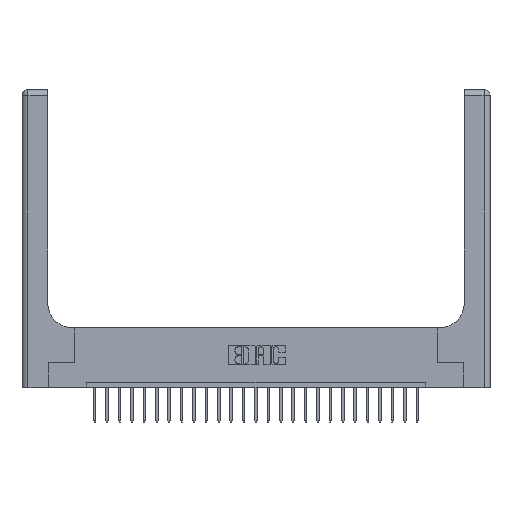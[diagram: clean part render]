
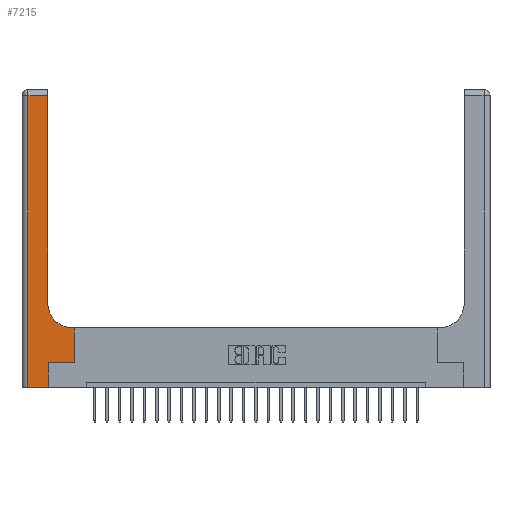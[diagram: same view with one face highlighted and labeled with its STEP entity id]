
A CAD part, top view. The second image highlights one B-rep face of the part: STEP entity #7215.
In plain terms, the highlighted planar face has unit normal (0, 0, 1).
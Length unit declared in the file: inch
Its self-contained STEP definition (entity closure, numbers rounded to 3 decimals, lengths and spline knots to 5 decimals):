
#197 = DIRECTION ( 'NONE',  ( 1., 0., 0. ) ) ;
#727 = EDGE_LOOP ( 'NONE', ( #18555, #17740, #23488, #21548, #5780, #23340, #6591, #14665, #17817 ) ) ;
#793 = DIRECTION ( 'NONE',  ( 0., 1., 0. ) ) ;
#932 = VECTOR ( 'NONE', #793, 39.37008 ) ;
#2665 = CARTESIAN_POINT ( 'NONE',  ( 0.265, 0., 0.37 ) ) ;
#2707 = AXIS2_PLACEMENT_3D ( 'NONE', #7221, #24271, #5247 ) ;
#3504 = DIRECTION ( 'NONE',  ( 0., 1., 0. ) ) ;
#3630 = LINE ( 'NONE', #18684, #20009 ) ;
#3648 = LINE ( 'NONE', #18702, #15636 ) ;
#4155 = LINE ( 'NONE', #9539, #5572 ) ;
#4341 = CARTESIAN_POINT ( 'NONE',  ( 0.06, 0., 0.37 ) ) ;
#5247 = DIRECTION ( 'NONE',  ( -1., 0., 0. ) ) ;
#5376 = EDGE_CURVE ( 'NONE', #9515, #13513, #16736, .T. ) ;
#5378 = LINE ( 'NONE', #12928, #6106 ) ;
#5572 = VECTOR ( 'NONE', #13419, 39.37008 ) ;
#5780 = ORIENTED_EDGE ( 'NONE', *, *, #15563, .T. ) ;
#6106 = VECTOR ( 'NONE', #20459, 39.37008 ) ;
#6144 = CARTESIAN_POINT ( 'NONE',  ( 0.06, 2.94, 0.37 ) ) ;
#6439 = VERTEX_POINT ( 'NONE', #6144 ) ;
#6472 = VERTEX_POINT ( 'NONE', #21458 ) ;
#6591 = ORIENTED_EDGE ( 'NONE', *, *, #5376, .T. ) ;
#6834 = CARTESIAN_POINT ( 'NONE',  ( 0.528, 0.25, 0.37 ) ) ;
#7151 = CARTESIAN_POINT ( 'NONE',  ( 0.528, 0.25, 0.37 ) ) ;
#7215 = ADVANCED_FACE ( 'NONE', ( #22198 ), #9039, .F. ) ;
#7221 = CARTESIAN_POINT ( 'NONE',  ( 0., 3., 0.37 ) ) ;
#7980 = VERTEX_POINT ( 'NONE', #16782 ) ;
#8187 = EDGE_CURVE ( 'NONE', #6439, #21183, #3648, .T. ) ;
#9039 = PLANE ( 'NONE',  #2707 ) ;
#9255 = DIRECTION ( 'NONE',  ( -1., 0., 0. ) ) ;
#9515 = VERTEX_POINT ( 'NONE', #7151 ) ;
#9539 = CARTESIAN_POINT ( 'NONE',  ( 0.26, 0.6, 0.37 ) ) ;
#9874 = VERTEX_POINT ( 'NONE', #18673 ) ;
#10772 = CARTESIAN_POINT ( 'NONE',  ( 0.26, 0.85, 0.37 ) ) ;
#11014 = LINE ( 'NONE', #16753, #17603 ) ;
#11211 = VERTEX_POINT ( 'NONE', #23532 ) ;
#11275 = VECTOR ( 'NONE', #3504, 39.37008 ) ;
#11291 = LINE ( 'NONE', #13051, #12152 ) ;
#12152 = VECTOR ( 'NONE', #197, 39.37008 ) ;
#12715 = DIRECTION ( 'NONE',  ( 1., 0., 0. ) ) ;
#12928 = CARTESIAN_POINT ( 'NONE',  ( 0.26, 3., 0.37 ) ) ;
#13051 = CARTESIAN_POINT ( 'NONE',  ( 0., 0., 0.37 ) ) ;
#13266 = DIRECTION ( 'NONE',  ( 1., 0., 0. ) ) ;
#13419 = DIRECTION ( 'NONE',  ( -1., 0., 0. ) ) ;
#13513 = VERTEX_POINT ( 'NONE', #13750 ) ;
#13750 = CARTESIAN_POINT ( 'NONE',  ( 0.528, 0.6, 0.37 ) ) ;
#14665 = ORIENTED_EDGE ( 'NONE', *, *, #14865, .T. ) ;
#14865 = EDGE_CURVE ( 'NONE', #13513, #9874, #4155, .T. ) ;
#15266 = DIRECTION ( 'NONE',  ( 0., 0., -1. ) ) ;
#15563 = EDGE_CURVE ( 'NONE', #11211, #7980, #18096, .T. ) ;
#15636 = VECTOR ( 'NONE', #17726, 39.37008 ) ;
#16347 = EDGE_CURVE ( 'NONE', #20302, #6472, #5378, .T. ) ;
#16355 = CIRCLE ( 'NONE', #19862, 0.25 ) ;
#16736 = LINE ( 'NONE', #6834, #11275 ) ;
#16753 = CARTESIAN_POINT ( 'NONE',  ( 0.265, 0.25, 0.37 ) ) ;
#16782 = CARTESIAN_POINT ( 'NONE',  ( 0.265, 0.25, 0.37 ) ) ;
#17603 = VECTOR ( 'NONE', #13266, 39.37008 ) ;
#17726 = DIRECTION ( 'NONE',  ( 0., -1., 0. ) ) ;
#17740 = ORIENTED_EDGE ( 'NONE', *, *, #20752, .T. ) ;
#17782 = EDGE_CURVE ( 'NONE', #7980, #9515, #11014, .T. ) ;
#17817 = ORIENTED_EDGE ( 'NONE', *, *, #21405, .T. ) ;
#18096 = LINE ( 'NONE', #2665, #932 ) ;
#18555 = ORIENTED_EDGE ( 'NONE', *, *, #16347, .T. ) ;
#18673 = CARTESIAN_POINT ( 'NONE',  ( 0.51, 0.6, 0.37 ) ) ;
#18684 = CARTESIAN_POINT ( 'NONE',  ( 0., 2.94, 0.37 ) ) ;
#18702 = CARTESIAN_POINT ( 'NONE',  ( 0.06, 3., 0.37 ) ) ;
#19862 = AXIS2_PLACEMENT_3D ( 'NONE', #20247, #15266, #12715 ) ;
#20009 = VECTOR ( 'NONE', #9255, 39.37008 ) ;
#20247 = CARTESIAN_POINT ( 'NONE',  ( 0.51, 0.85, 0.37 ) ) ;
#20302 = VERTEX_POINT ( 'NONE', #10772 ) ;
#20459 = DIRECTION ( 'NONE',  ( 0., 1., 0. ) ) ;
#20752 = EDGE_CURVE ( 'NONE', #6472, #6439, #3630, .T. ) ;
#21183 = VERTEX_POINT ( 'NONE', #4341 ) ;
#21405 = EDGE_CURVE ( 'NONE', #9874, #20302, #16355, .T. ) ;
#21458 = CARTESIAN_POINT ( 'NONE',  ( 0.26, 2.94, 0.37 ) ) ;
#21548 = ORIENTED_EDGE ( 'NONE', *, *, #23964, .T. ) ;
#22198 = FACE_OUTER_BOUND ( 'NONE', #727, .T. ) ;
#23340 = ORIENTED_EDGE ( 'NONE', *, *, #17782, .T. ) ;
#23488 = ORIENTED_EDGE ( 'NONE', *, *, #8187, .T. ) ;
#23532 = CARTESIAN_POINT ( 'NONE',  ( 0.265, 0., 0.37 ) ) ;
#23964 = EDGE_CURVE ( 'NONE', #21183, #11211, #11291, .T. ) ;
#24271 = DIRECTION ( 'NONE',  ( 0., 0., -1. ) ) ;
